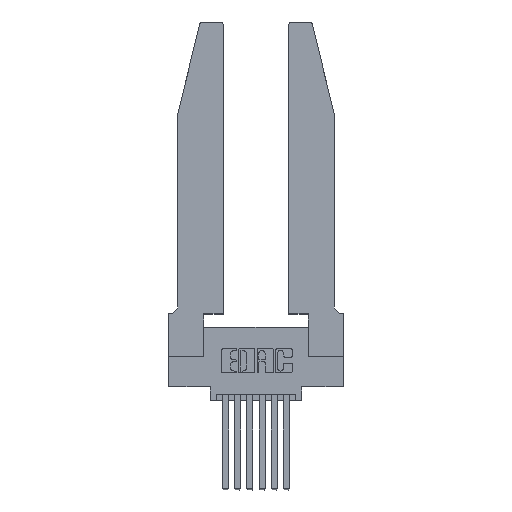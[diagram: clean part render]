
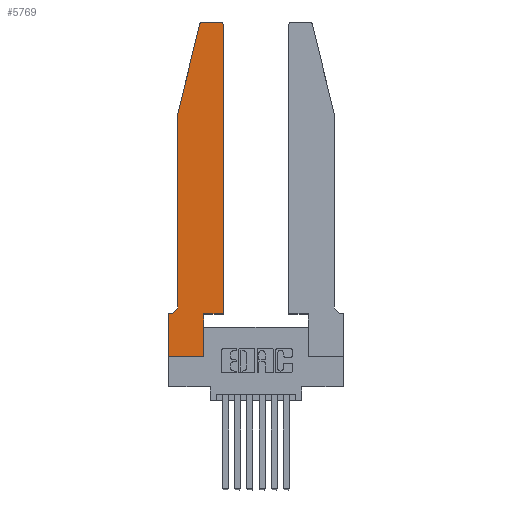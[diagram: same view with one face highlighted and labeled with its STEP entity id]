
A CAD part, top view. The second image highlights one B-rep face of the part: STEP entity #5769.
In plain terms, the highlighted planar face has unit normal (0, 0, 1).
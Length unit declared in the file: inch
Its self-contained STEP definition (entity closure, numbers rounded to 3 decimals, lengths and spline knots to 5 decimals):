
#222 = CARTESIAN_POINT ( 'NONE',  ( 0., 0., 0.37 ) ) ;
#349 = DIRECTION ( 'NONE',  ( 1., 0., 0. ) ) ;
#424 = CARTESIAN_POINT ( 'NONE',  ( 0.2865, 0., 0.37 ) ) ;
#480 = DIRECTION ( 'NONE',  ( 1., 0., 0. ) ) ;
#914 = LINE ( 'NONE', #2581, #9558 ) ;
#977 = CARTESIAN_POINT ( 'NONE',  ( 0.2865, 0.35, 0.37 ) ) ;
#1100 = EDGE_CURVE ( 'NONE', #3117, #5242, #6745, .T. ) ;
#1104 = CARTESIAN_POINT ( 'NONE',  ( 0., 0., 0.37 ) ) ;
#1120 = CARTESIAN_POINT ( 'NONE',  ( 0., 0.35, 0.37 ) ) ;
#1266 = ORIENTED_EDGE ( 'NONE', *, *, #9284, .T. ) ;
#1476 = VECTOR ( 'NONE', #10634, 39.37008 ) ;
#1494 = VERTEX_POINT ( 'NONE', #11344 ) ;
#1725 = DIRECTION ( 'NONE',  ( -0.239, -0.971, 0. ) ) ;
#1742 = VERTEX_POINT ( 'NONE', #4985 ) ;
#2004 = PLANE ( 'NONE',  #13619 ) ;
#2039 = CARTESIAN_POINT ( 'NONE',  ( 0.284, 2.75, 0.37 ) ) ;
#2055 = ORIENTED_EDGE ( 'NONE', *, *, #12315, .T. ) ;
#2120 = EDGE_CURVE ( 'NONE', #6638, #3117, #7075, .T. ) ;
#2142 = EDGE_LOOP ( 'NONE', ( #8229, #5843, #13366, #2055, #8804, #13404, #2308, #6618, #9214, #1266, #6804, #12996 ) ) ;
#2308 = ORIENTED_EDGE ( 'NONE', *, *, #5637, .T. ) ;
#2581 = CARTESIAN_POINT ( 'NONE',  ( 0.2605, 2.75, 0.37 ) ) ;
#2685 = CARTESIAN_POINT ( 'NONE',  ( 0.4505, 0.35, 0.37 ) ) ;
#3051 = EDGE_CURVE ( 'NONE', #7499, #7872, #8760, .T. ) ;
#3117 = VERTEX_POINT ( 'NONE', #424 ) ;
#3179 = DIRECTION ( 'NONE',  ( 1., 0., 0. ) ) ;
#3204 = EDGE_CURVE ( 'NONE', #11172, #1742, #7045, .T. ) ;
#3787 = VECTOR ( 'NONE', #6187, 39.37008 ) ;
#3866 = DIRECTION ( 'NONE',  ( 1., 0., 0. ) ) ;
#4117 = VECTOR ( 'NONE', #480, 39.37008 ) ;
#4370 = CARTESIAN_POINT ( 'NONE',  ( 0.25487, 2.72718, 0.37 ) ) ;
#4384 = AXIS2_PLACEMENT_3D ( 'NONE', #13526, #7223, #349 ) ;
#4955 = CARTESIAN_POINT ( 'NONE',  ( 0.0755, 0.35, 0.37 ) ) ;
#4985 = CARTESIAN_POINT ( 'NONE',  ( 0.0755, 2., 0.37 ) ) ;
#5033 = CARTESIAN_POINT ( 'NONE',  ( 0.4505, 0.35, 0.37 ) ) ;
#5091 = VERTEX_POINT ( 'NONE', #6502 ) ;
#5098 = CARTESIAN_POINT ( 'NONE',  ( 0.4505, 0.35, 0.37 ) ) ;
#5154 = CARTESIAN_POINT ( 'NONE',  ( 0.0755, 2., 0.37 ) ) ;
#5242 = VERTEX_POINT ( 'NONE', #10004 ) ;
#5355 = CARTESIAN_POINT ( 'NONE',  ( 0.0055, 0.42, 0.37 ) ) ;
#5416 = AXIS2_PLACEMENT_3D ( 'NONE', #5503, #12960, #6617 ) ;
#5451 = EDGE_CURVE ( 'NONE', #1494, #13108, #914, .T. ) ;
#5503 = CARTESIAN_POINT ( 'NONE',  ( 0.284, 2.72, 0.37 ) ) ;
#5637 = EDGE_CURVE ( 'NONE', #7872, #6638, #7555, .T. ) ;
#5769 = ADVANCED_FACE ( 'NONE', ( #9386 ), #2004, .T. ) ;
#5843 = ORIENTED_EDGE ( 'NONE', *, *, #14135, .T. ) ;
#5960 = CIRCLE ( 'NONE', #5416, 0.03 ) ;
#6057 = AXIS2_PLACEMENT_3D ( 'NONE', #5355, #12828, #6480 ) ;
#6187 = DIRECTION ( 'NONE',  ( 0., 1., 0. ) ) ;
#6243 = CARTESIAN_POINT ( 'NONE',  ( 0.0055, 0.35, 0.37 ) ) ;
#6480 = DIRECTION ( 'NONE',  ( -1., 0., 0. ) ) ;
#6502 = CARTESIAN_POINT ( 'NONE',  ( 0.0755, 0.42, 0.37 ) ) ;
#6617 = DIRECTION ( 'NONE',  ( 1., 0., 0. ) ) ;
#6618 = ORIENTED_EDGE ( 'NONE', *, *, #2120, .T. ) ;
#6638 = VERTEX_POINT ( 'NONE', #1104 ) ;
#6680 = CIRCLE ( 'NONE', #6057, 0.07 ) ;
#6745 = LINE ( 'NONE', #977, #3787 ) ;
#6804 = ORIENTED_EDGE ( 'NONE', *, *, #8547, .T. ) ;
#7045 = LINE ( 'NONE', #5154, #9586 ) ;
#7071 = DIRECTION ( 'NONE',  ( -1., 0., 0. ) ) ;
#7075 = LINE ( 'NONE', #222, #4117 ) ;
#7168 = VERTEX_POINT ( 'NONE', #10026 ) ;
#7223 = DIRECTION ( 'NONE',  ( 0., 0., 1. ) ) ;
#7499 = VERTEX_POINT ( 'NONE', #6243 ) ;
#7555 = LINE ( 'NONE', #11654, #1476 ) ;
#7872 = VERTEX_POINT ( 'NONE', #1120 ) ;
#7916 = LINE ( 'NONE', #10034, #13485 ) ;
#8229 = ORIENTED_EDGE ( 'NONE', *, *, #5451, .T. ) ;
#8547 = EDGE_CURVE ( 'NONE', #13501, #7168, #10979, .T. ) ;
#8760 = LINE ( 'NONE', #4955, #11235 ) ;
#8804 = ORIENTED_EDGE ( 'NONE', *, *, #12659, .T. ) ;
#9214 = ORIENTED_EDGE ( 'NONE', *, *, #1100, .T. ) ;
#9284 = EDGE_CURVE ( 'NONE', #5242, #13501, #10479, .T. ) ;
#9386 = FACE_OUTER_BOUND ( 'NONE', #2142, .T. ) ;
#9558 = VECTOR ( 'NONE', #7071, 39.37008 ) ;
#9586 = VECTOR ( 'NONE', #1725, 39.37008 ) ;
#9789 = EDGE_CURVE ( 'NONE', #7168, #1494, #12560, .T. ) ;
#9807 = DIRECTION ( 'NONE',  ( 0., 0., 1. ) ) ;
#10004 = CARTESIAN_POINT ( 'NONE',  ( 0.2865, 0.35, 0.37 ) ) ;
#10026 = CARTESIAN_POINT ( 'NONE',  ( 0.4505, 2.72, 0.37 ) ) ;
#10034 = CARTESIAN_POINT ( 'NONE',  ( 0.0755, 2., 0.37 ) ) ;
#10479 = LINE ( 'NONE', #2685, #12890 ) ;
#10634 = DIRECTION ( 'NONE',  ( 0., -1., 0. ) ) ;
#10979 = LINE ( 'NONE', #5033, #12756 ) ;
#11085 = DIRECTION ( 'NONE',  ( 0., -1., 0. ) ) ;
#11172 = VERTEX_POINT ( 'NONE', #4370 ) ;
#11235 = VECTOR ( 'NONE', #13503, 39.37008 ) ;
#11344 = CARTESIAN_POINT ( 'NONE',  ( 0.4205, 2.75, 0.37 ) ) ;
#11654 = CARTESIAN_POINT ( 'NONE',  ( 0., 0., 0.37 ) ) ;
#12315 = EDGE_CURVE ( 'NONE', #1742, #5091, #7916, .T. ) ;
#12532 = DIRECTION ( 'NONE',  ( 0., 1., 0. ) ) ;
#12560 = CIRCLE ( 'NONE', #4384, 0.03 ) ;
#12659 = EDGE_CURVE ( 'NONE', #5091, #7499, #6680, .T. ) ;
#12756 = VECTOR ( 'NONE', #12532, 39.37008 ) ;
#12828 = DIRECTION ( 'NONE',  ( 0., 0., -1. ) ) ;
#12890 = VECTOR ( 'NONE', #3866, 39.37008 ) ;
#12960 = DIRECTION ( 'NONE',  ( 0., 0., 1. ) ) ;
#12996 = ORIENTED_EDGE ( 'NONE', *, *, #9789, .T. ) ;
#13108 = VERTEX_POINT ( 'NONE', #2039 ) ;
#13366 = ORIENTED_EDGE ( 'NONE', *, *, #3204, .T. ) ;
#13404 = ORIENTED_EDGE ( 'NONE', *, *, #3051, .T. ) ;
#13485 = VECTOR ( 'NONE', #11085, 39.37008 ) ;
#13501 = VERTEX_POINT ( 'NONE', #5098 ) ;
#13503 = DIRECTION ( 'NONE',  ( -1., 0., 0. ) ) ;
#13526 = CARTESIAN_POINT ( 'NONE',  ( 0.4205, 2.72, 0.37 ) ) ;
#13619 = AXIS2_PLACEMENT_3D ( 'NONE', #13946, #9807, #3179 ) ;
#13946 = CARTESIAN_POINT ( 'NONE',  ( 0., 0.35, 0.37 ) ) ;
#14135 = EDGE_CURVE ( 'NONE', #13108, #11172, #5960, .T. ) ;
